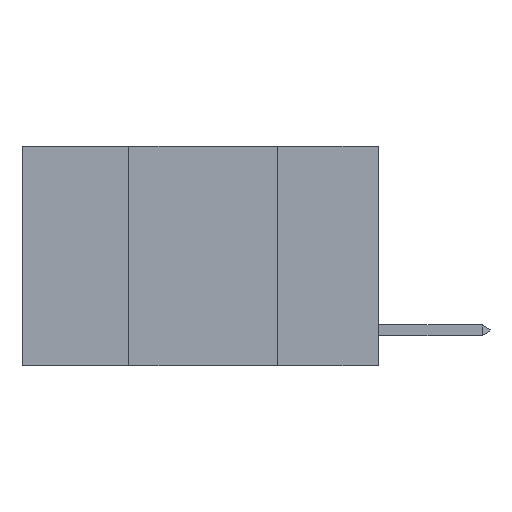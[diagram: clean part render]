
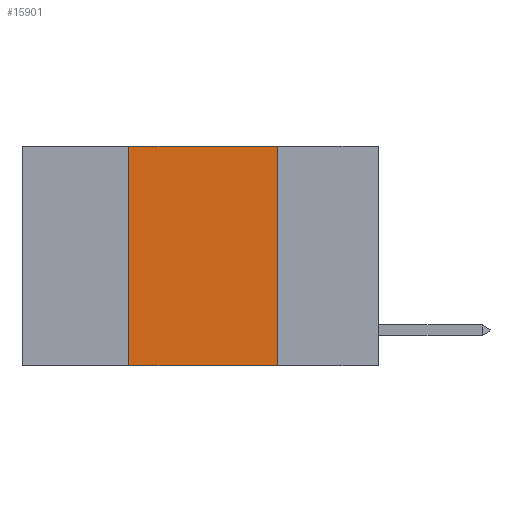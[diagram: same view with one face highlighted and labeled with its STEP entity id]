
A CAD part, left-side view. The second image highlights one B-rep face of the part: STEP entity #15901.
In plain terms, the highlighted planar face has unit normal (-1, 0, 0).
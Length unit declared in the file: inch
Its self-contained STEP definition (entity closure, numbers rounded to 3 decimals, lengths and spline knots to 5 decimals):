
#820 = EDGE_LOOP ( 'NONE', ( #13895, #4009, #1952, #19325 ) ) ;
#1179 = VERTEX_POINT ( 'NONE', #19823 ) ;
#1387 = FACE_OUTER_BOUND ( 'NONE', #820, .T. ) ;
#1512 = EDGE_CURVE ( 'NONE', #21426, #18351, #16224, .T. ) ;
#1952 = ORIENTED_EDGE ( 'NONE', *, *, #15214, .F. ) ;
#1990 = VECTOR ( 'NONE', #21870, 39.37008 ) ;
#2304 = CARTESIAN_POINT ( 'NONE',  ( 0., 0.6, 0. ) ) ;
#2361 = DIRECTION ( 'NONE',  ( 0., 0., -1. ) ) ;
#2476 = DIRECTION ( 'NONE',  ( 0., -1., 0. ) ) ;
#2800 = LINE ( 'NONE', #5357, #16500 ) ;
#3025 = VECTOR ( 'NONE', #2361, 39.37008 ) ;
#3405 = EDGE_CURVE ( 'NONE', #18351, #1179, #17295, .T. ) ;
#4009 = ORIENTED_EDGE ( 'NONE', *, *, #1512, .F. ) ;
#4072 = DIRECTION ( 'NONE',  ( 0., 0., -1. ) ) ;
#4969 = CARTESIAN_POINT ( 'NONE',  ( 0., 0.17, 0. ) ) ;
#5357 = CARTESIAN_POINT ( 'NONE',  ( 0., 0.42, 0. ) ) ;
#5374 = LINE ( 'NONE', #13163, #19092 ) ;
#8963 = DIRECTION ( 'NONE',  ( 0., 0., 1. ) ) ;
#9193 = VERTEX_POINT ( 'NONE', #11669 ) ;
#9980 = AXIS2_PLACEMENT_3D ( 'NONE', #2304, #14804, #4072 ) ;
#11154 = CARTESIAN_POINT ( 'NONE',  ( 0., 0.6, 0. ) ) ;
#11245 = CARTESIAN_POINT ( 'NONE',  ( 0., 0.17, 0. ) ) ;
#11669 = CARTESIAN_POINT ( 'NONE',  ( 0., 0.42, -0.37 ) ) ;
#13163 = CARTESIAN_POINT ( 'NONE',  ( 0., 0.6, -0.37 ) ) ;
#13895 = ORIENTED_EDGE ( 'NONE', *, *, #3405, .F. ) ;
#14017 = EDGE_CURVE ( 'NONE', #9193, #1179, #5374, .T. ) ;
#14804 = DIRECTION ( 'NONE',  ( 1., 0., 0. ) ) ;
#15214 = EDGE_CURVE ( 'NONE', #9193, #21426, #2800, .T. ) ;
#15544 = CARTESIAN_POINT ( 'NONE',  ( 0., 0.42, 0. ) ) ;
#15901 = ADVANCED_FACE ( 'NONE', ( #1387 ), #20110, .F. ) ;
#16224 = LINE ( 'NONE', #11154, #1990 ) ;
#16500 = VECTOR ( 'NONE', #8963, 39.37008 ) ;
#17295 = LINE ( 'NONE', #11245, #3025 ) ;
#18351 = VERTEX_POINT ( 'NONE', #4969 ) ;
#19092 = VECTOR ( 'NONE', #2476, 39.37008 ) ;
#19325 = ORIENTED_EDGE ( 'NONE', *, *, #14017, .T. ) ;
#19823 = CARTESIAN_POINT ( 'NONE',  ( 0., 0.17, -0.37 ) ) ;
#20110 = PLANE ( 'NONE',  #9980 ) ;
#21426 = VERTEX_POINT ( 'NONE', #15544 ) ;
#21870 = DIRECTION ( 'NONE',  ( 0., -1., 0. ) ) ;
